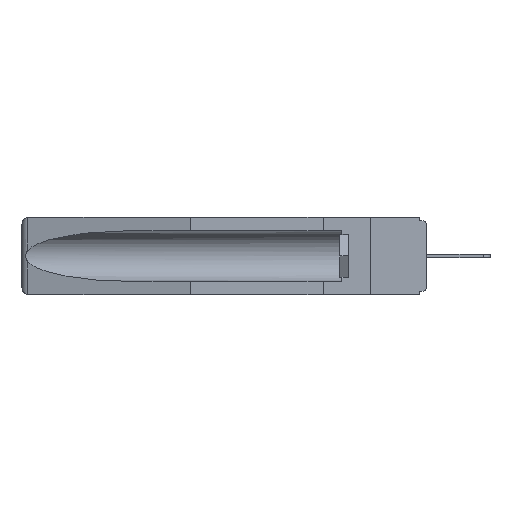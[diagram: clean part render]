
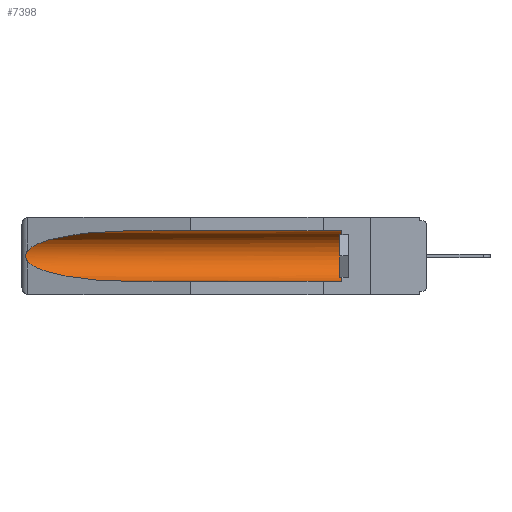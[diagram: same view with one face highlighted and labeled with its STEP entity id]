
A CAD part, left-side view. The second image highlights one B-rep face of the part: STEP entity #7398.
In plain terms, the highlighted cylindrical face has radius 2.857 mm (diameter 5.715 mm), a partial arc.
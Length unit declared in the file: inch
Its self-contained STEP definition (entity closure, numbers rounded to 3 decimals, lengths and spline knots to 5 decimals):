
#345 = CARTESIAN_POINT ( 'NONE',  ( 0.155, 1.07973, -0.059 ) ) ;
#879 = DIRECTION ( 'NONE',  ( 0., 0., 1. ) ) ;
#958 = VECTOR ( 'NONE', #5678, 39.37008 ) ;
#1198 = DIRECTION ( 'NONE',  ( 0., 1., 0. ) ) ;
#1257 = CARTESIAN_POINT ( 'NONE',  ( 0.155, -0.30754, -0.059 ) ) ;
#1410 = LINE ( 'NONE', #1257, #958 ) ;
#2012 = CARTESIAN_POINT ( 'NONE',  ( 0.155, 1.07973, -0.284 ) ) ;
#2296 = CARTESIAN_POINT ( 'NONE',  ( 0.155, -0.30754, -0.1715 ) ) ;
#2547 = CARTESIAN_POINT ( 'NONE',  ( 0.2673, 1.5327, -0.16383 ) ) ;
#2632 = AXIS2_PLACEMENT_3D ( 'NONE', #2296, #18002, #879 ) ;
#3311 = CARTESIAN_POINT ( 'NONE',  ( 0.26537, 1.52718, -0.14972 ) ) ;
#3312 = ORIENTED_EDGE ( 'NONE', *, *, #6050, .T. ) ;
#4033 = CARTESIAN_POINT ( 'NONE',  ( 0.2675, 1.53308, -0.17534 ) ) ;
#4229 = ORIENTED_EDGE ( 'NONE', *, *, #12716, .T. ) ;
#4420 = B_SPLINE_CURVE_WITH_KNOTS ( 'NONE', 3,
 ( #6906, #18172, #11230, #2547, #12601, #4033, #14007, #5503, #15453, #6961 ),
 .UNSPECIFIED., .F., .F.,
 ( 4, 2, 2, 2, 4 ),
 ( 0., 0.00029, 0.00058, 0.00087, 0.00117 ),
 .UNSPECIFIED. ) ;
#4840 = LINE ( 'NONE', #18276, #15756 ) ;
#4989 = VERTEX_POINT ( 'NONE', #18156 ) ;
#5239 =( BOUNDED_CURVE ( )  B_SPLINE_CURVE ( 3, ( #9412, #7190, #8146, #8109 ),
 .UNSPECIFIED., .F., .F. ) 
 B_SPLINE_CURVE_WITH_KNOTS ( ( 4, 4 ),
 ( 0.1948, 1.5708 ),
 .UNSPECIFIED. ) 
 CURVE ( )  GEOMETRIC_REPRESENTATION_ITEM ( )  RATIONAL_B_SPLINE_CURVE ( ( 1., 0.848, 0.848, 1. ) ) 
 REPRESENTATION_ITEM ( '' )  );
#5445 = EDGE_LOOP ( 'NONE', ( #16706, #6289, #3312, #11033, #15187, #4229 ) ) ;
#5503 = CARTESIAN_POINT ( 'NONE',  ( 0.26655, 1.53094, -0.18657 ) ) ;
#5678 = DIRECTION ( 'NONE',  ( 0., 1., 0. ) ) ;
#5741 = CARTESIAN_POINT ( 'NONE',  ( 0.155, 0.126, -0.284 ) ) ;
#6050 = EDGE_CURVE ( 'NONE', #4989, #12091, #5239, .T. ) ;
#6289 = ORIENTED_EDGE ( 'NONE', *, *, #12607, .T. ) ;
#6906 = CARTESIAN_POINT ( 'NONE',  ( 0.26537, 1.52718, -0.14972 ) ) ;
#6961 = CARTESIAN_POINT ( 'NONE',  ( 0.26537, 1.52718, -0.19328 ) ) ;
#7190 = CARTESIAN_POINT ( 'NONE',  ( 0.25451, 1.48313, -0.24835 ) ) ;
#7398 = ADVANCED_FACE ( 'NONE', ( #11424 ), #11011, .F. ) ;
#7927 = CARTESIAN_POINT ( 'NONE',  ( 0.155, 0.126, -0.1715 ) ) ;
#8109 = CARTESIAN_POINT ( 'NONE',  ( 0.155, 1.07973, -0.284 ) ) ;
#8146 = CARTESIAN_POINT ( 'NONE',  ( 0.21114, 1.30732, -0.284 ) ) ;
#8872 = EDGE_CURVE ( 'NONE', #9934, #12091, #4840, .T. ) ;
#8902 = VERTEX_POINT ( 'NONE', #14189 ) ;
#9151 = CARTESIAN_POINT ( 'NONE',  ( 0.21114, 1.30732, -0.059 ) ) ;
#9412 = CARTESIAN_POINT ( 'NONE',  ( 0.26537, 1.52718, -0.19328 ) ) ;
#9456 = DIRECTION ( 'NONE',  ( 0., 0., 1. ) ) ;
#9934 = VERTEX_POINT ( 'NONE', #5741 ) ;
#10855 = CARTESIAN_POINT ( 'NONE',  ( 0.155, 1.07973, -0.059 ) ) ;
#10879 = VERTEX_POINT ( 'NONE', #12212 ) ;
#11011 = CYLINDRICAL_SURFACE ( 'NONE', #2632, 0.1125 ) ;
#11033 = ORIENTED_EDGE ( 'NONE', *, *, #8872, .F. ) ;
#11230 = CARTESIAN_POINT ( 'NONE',  ( 0.26654, 1.53092, -0.15636 ) ) ;
#11243 =( BOUNDED_CURVE ( )  B_SPLINE_CURVE ( 3, ( #345, #9151, #11933, #3311 ),
 .UNSPECIFIED., .F., .F. ) 
 B_SPLINE_CURVE_WITH_KNOTS ( ( 4, 4 ),
 ( 4.71239, 6.08839 ),
 .UNSPECIFIED. ) 
 CURVE ( )  GEOMETRIC_REPRESENTATION_ITEM ( )  RATIONAL_B_SPLINE_CURVE ( ( 1., 0.848, 0.848, 1. ) ) 
 REPRESENTATION_ITEM ( '' )  );
#11424 = FACE_OUTER_BOUND ( 'NONE', #5445, .T. ) ;
#11545 = AXIS2_PLACEMENT_3D ( 'NONE', #7927, #17809, #9456 ) ;
#11933 = CARTESIAN_POINT ( 'NONE',  ( 0.25451, 1.48313, -0.09465 ) ) ;
#12091 = VERTEX_POINT ( 'NONE', #2012 ) ;
#12212 = CARTESIAN_POINT ( 'NONE',  ( 0.155, 0.126, -0.059 ) ) ;
#12601 = CARTESIAN_POINT ( 'NONE',  ( 0.2675, 1.53308, -0.16763 ) ) ;
#12607 = EDGE_CURVE ( 'NONE', #8902, #4989, #4420, .T. ) ;
#12716 = EDGE_CURVE ( 'NONE', #10879, #15901, #1410, .T. ) ;
#12949 = EDGE_CURVE ( 'NONE', #15901, #8902, #11243, .T. ) ;
#13552 = EDGE_CURVE ( 'NONE', #9934, #10879, #17048, .T. ) ;
#14007 = CARTESIAN_POINT ( 'NONE',  ( 0.2673, 1.53269, -0.17917 ) ) ;
#14189 = CARTESIAN_POINT ( 'NONE',  ( 0.26537, 1.52718, -0.14972 ) ) ;
#15187 = ORIENTED_EDGE ( 'NONE', *, *, #13552, .T. ) ;
#15453 = CARTESIAN_POINT ( 'NONE',  ( 0.26597, 1.5296, -0.19026 ) ) ;
#15756 = VECTOR ( 'NONE', #1198, 39.37008 ) ;
#15901 = VERTEX_POINT ( 'NONE', #10855 ) ;
#16706 = ORIENTED_EDGE ( 'NONE', *, *, #12949, .T. ) ;
#17048 = CIRCLE ( 'NONE', #11545, 0.1125 ) ;
#17809 = DIRECTION ( 'NONE',  ( 0., -1., 0. ) ) ;
#18002 = DIRECTION ( 'NONE',  ( 0., 1., 0. ) ) ;
#18156 = CARTESIAN_POINT ( 'NONE',  ( 0.26537, 1.52718, -0.19328 ) ) ;
#18172 = CARTESIAN_POINT ( 'NONE',  ( 0.26597, 1.52961, -0.15275 ) ) ;
#18276 = CARTESIAN_POINT ( 'NONE',  ( 0.155, -0.30754, -0.284 ) ) ;
